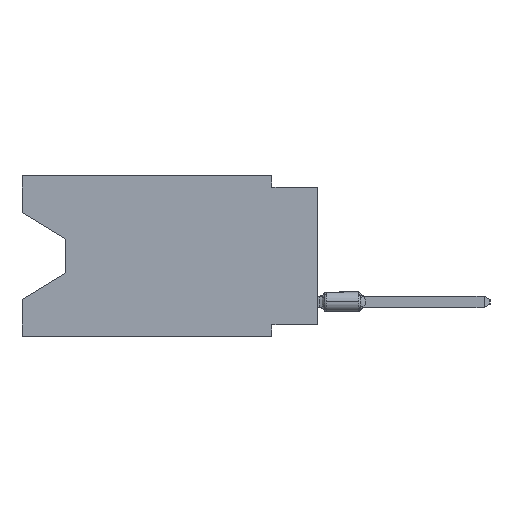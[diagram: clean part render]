
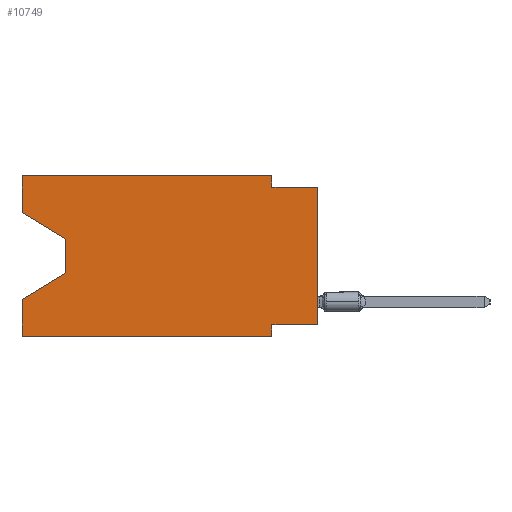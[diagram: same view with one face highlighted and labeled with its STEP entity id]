
A CAD part, left-side view. The second image highlights one B-rep face of the part: STEP entity #10749.
In plain terms, the highlighted planar face has unit normal (-1, 0, 0).
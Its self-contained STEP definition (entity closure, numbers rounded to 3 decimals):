
#308 = VERTEX_POINT ( 'NONE', #32423 ) ;
#1716 = ORIENTED_EDGE ( 'NONE', *, *, #21301, .T. ) ;
#2599 = VECTOR ( 'NONE', #13432, 1000. ) ;
#2848 = DIRECTION ( 'NONE',  ( 0., -1., 0. ) ) ;
#2854 = FACE_OUTER_BOUND ( 'NONE', #40116, .T. ) ;
#3252 = VERTEX_POINT ( 'NONE', #16704 ) ;
#3814 = CARTESIAN_POINT ( 'NONE',  ( 0., 2.54, -0.635 ) ) ;
#4680 = VECTOR ( 'NONE', #42543, 1000. ) ;
#5676 = VECTOR ( 'NONE', #6606, 1000. ) ;
#6606 = DIRECTION ( 'NONE',  ( 0., 0., -1. ) ) ;
#7299 = CARTESIAN_POINT ( 'NONE',  ( 0., 13.97, -3.505 ) ) ;
#7644 = CARTESIAN_POINT ( 'NONE',  ( 0., 16.383, 0. ) ) ;
#8144 = EDGE_CURVE ( 'NONE', #308, #26941, #40598, .T. ) ;
#8323 = CARTESIAN_POINT ( 'NONE',  ( 0., 16.383, -2.038 ) ) ;
#8617 = EDGE_CURVE ( 'NONE', #10358, #3252, #24710, .T. ) ;
#10027 = CARTESIAN_POINT ( 'NONE',  ( 0., 16.383, 0. ) ) ;
#10358 = VERTEX_POINT ( 'NONE', #16991 ) ;
#10749 = ADVANCED_FACE ( 'NONE', ( #2854 ), #16099, .F. ) ;
#10778 = LINE ( 'NONE', #16878, #35163 ) ;
#11109 = VECTOR ( 'NONE', #17625, 1000. ) ;
#11464 = ORIENTED_EDGE ( 'NONE', *, *, #41612, .F. ) ;
#11743 = VECTOR ( 'NONE', #32969, 1000. ) ;
#12427 = EDGE_CURVE ( 'NONE', #31995, #13780, #22536, .T. ) ;
#12822 = DIRECTION ( 'NONE',  ( 1., 0., 0. ) ) ;
#13432 = DIRECTION ( 'NONE',  ( 0., 1., 0. ) ) ;
#13780 = VERTEX_POINT ( 'NONE', #7299 ) ;
#14572 = ORIENTED_EDGE ( 'NONE', *, *, #26797, .T. ) ;
#15048 = LINE ( 'NONE', #21340, #22914 ) ;
#16099 = PLANE ( 'NONE',  #25712 ) ;
#16292 = CARTESIAN_POINT ( 'NONE',  ( 0., 16.383, -8.89 ) ) ;
#16387 = CARTESIAN_POINT ( 'NONE',  ( 0., 2.54, -8.89 ) ) ;
#16704 = CARTESIAN_POINT ( 'NONE',  ( 0., 16.383, -6.852 ) ) ;
#16878 = CARTESIAN_POINT ( 'NONE',  ( 0., 13.97, -5.385 ) ) ;
#16991 = CARTESIAN_POINT ( 'NONE',  ( 0., 16.383, -8.89 ) ) ;
#17625 = DIRECTION ( 'NONE',  ( 0., -1., 0. ) ) ;
#17955 = LINE ( 'NONE', #27698, #40091 ) ;
#18633 = VECTOR ( 'NONE', #34685, 1000. ) ;
#18640 = CARTESIAN_POINT ( 'NONE',  ( 0., 16.383, 0. ) ) ;
#19757 = LINE ( 'NONE', #16292, #11743 ) ;
#19933 = LINE ( 'NONE', #29273, #2599 ) ;
#20316 = CARTESIAN_POINT ( 'NONE',  ( 0., 0., -8.255 ) ) ;
#20758 = DIRECTION ( 'NONE',  ( 0., 0.855, -0.519 ) ) ;
#21301 = EDGE_CURVE ( 'NONE', #13780, #37296, #17955, .T. ) ;
#21340 = CARTESIAN_POINT ( 'NONE',  ( 0., 0., 0. ) ) ;
#21455 = CARTESIAN_POINT ( 'NONE',  ( 0., 2.54, 0. ) ) ;
#21619 = VERTEX_POINT ( 'NONE', #3814 ) ;
#22292 = VECTOR ( 'NONE', #35880, 1000. ) ;
#22536 = LINE ( 'NONE', #42030, #31858 ) ;
#22914 = VECTOR ( 'NONE', #34560, 1000. ) ;
#23104 = LINE ( 'NONE', #39782, #22292 ) ;
#23273 = EDGE_CURVE ( 'NONE', #30101, #32927, #23104, .T. ) ;
#24710 = LINE ( 'NONE', #18640, #18633 ) ;
#25712 = AXIS2_PLACEMENT_3D ( 'NONE', #29312, #12822, #26054 ) ;
#25946 = ORIENTED_EDGE ( 'NONE', *, *, #8617, .F. ) ;
#26054 = DIRECTION ( 'NONE',  ( 0., 0., -1. ) ) ;
#26562 = LINE ( 'NONE', #40206, #5676 ) ;
#26771 = EDGE_CURVE ( 'NONE', #21619, #27890, #36440, .T. ) ;
#26797 = EDGE_CURVE ( 'NONE', #10358, #32927, #19757, .T. ) ;
#26941 = VERTEX_POINT ( 'NONE', #21455 ) ;
#27295 = DIRECTION ( 'NONE',  ( 0., 0., -1. ) ) ;
#27652 = VECTOR ( 'NONE', #2848, 1000. ) ;
#27698 = CARTESIAN_POINT ( 'NONE',  ( 0., 13.97, -3.505 ) ) ;
#27809 = EDGE_CURVE ( 'NONE', #40372, #27890, #15048, .T. ) ;
#27890 = VERTEX_POINT ( 'NONE', #32612 ) ;
#29181 = ORIENTED_EDGE ( 'NONE', *, *, #12427, .T. ) ;
#29273 = CARTESIAN_POINT ( 'NONE',  ( 0., 0., -8.255 ) ) ;
#29312 = CARTESIAN_POINT ( 'NONE',  ( 0., 16.383, 0. ) ) ;
#29572 = ORIENTED_EDGE ( 'NONE', *, *, #27809, .T. ) ;
#29667 = ORIENTED_EDGE ( 'NONE', *, *, #40228, .F. ) ;
#29737 = ORIENTED_EDGE ( 'NONE', *, *, #8144, .F. ) ;
#30101 = VERTEX_POINT ( 'NONE', #35951 ) ;
#30134 = EDGE_CURVE ( 'NONE', #37296, #3252, #10778, .T. ) ;
#30141 = ORIENTED_EDGE ( 'NONE', *, *, #30134, .T. ) ;
#31787 = ORIENTED_EDGE ( 'NONE', *, *, #23273, .F. ) ;
#31858 = VECTOR ( 'NONE', #38794, 1000. ) ;
#31981 = CARTESIAN_POINT ( 'NONE',  ( 0., 13.97, -5.385 ) ) ;
#31995 = VERTEX_POINT ( 'NONE', #8323 ) ;
#32423 = CARTESIAN_POINT ( 'NONE',  ( 0., 16.383, 0. ) ) ;
#32612 = CARTESIAN_POINT ( 'NONE',  ( 0., 0., -0.635 ) ) ;
#32927 = VERTEX_POINT ( 'NONE', #16387 ) ;
#32969 = DIRECTION ( 'NONE',  ( 0., -1., 0. ) ) ;
#33688 = ORIENTED_EDGE ( 'NONE', *, *, #26771, .F. ) ;
#34560 = DIRECTION ( 'NONE',  ( 0., 0., 1. ) ) ;
#34685 = DIRECTION ( 'NONE',  ( 0., 0., 1. ) ) ;
#34999 = ORIENTED_EDGE ( 'NONE', *, *, #38636, .F. ) ;
#35163 = VECTOR ( 'NONE', #20758, 1000. ) ;
#35880 = DIRECTION ( 'NONE',  ( 0., 0., -1. ) ) ;
#35951 = CARTESIAN_POINT ( 'NONE',  ( 0., 2.54, -8.255 ) ) ;
#36012 = CARTESIAN_POINT ( 'NONE',  ( 0., 0., -0.635 ) ) ;
#36440 = LINE ( 'NONE', #36012, #27652 ) ;
#37296 = VERTEX_POINT ( 'NONE', #31981 ) ;
#38636 = EDGE_CURVE ( 'NONE', #26941, #21619, #26562, .T. ) ;
#38794 = DIRECTION ( 'NONE',  ( 0., -0.855, -0.519 ) ) ;
#39731 = LINE ( 'NONE', #10027, #4680 ) ;
#39782 = CARTESIAN_POINT ( 'NONE',  ( 0., 2.54, -8.89 ) ) ;
#40091 = VECTOR ( 'NONE', #27295, 1000. ) ;
#40116 = EDGE_LOOP ( 'NONE', ( #29181, #1716, #30141, #25946, #14572, #31787, #11464, #29572, #33688, #34999, #29737, #29667 ) ) ;
#40206 = CARTESIAN_POINT ( 'NONE',  ( 0., 2.54, 0. ) ) ;
#40228 = EDGE_CURVE ( 'NONE', #31995, #308, #39731, .T. ) ;
#40372 = VERTEX_POINT ( 'NONE', #20316 ) ;
#40598 = LINE ( 'NONE', #7644, #11109 ) ;
#41612 = EDGE_CURVE ( 'NONE', #40372, #30101, #19933, .T. ) ;
#42030 = CARTESIAN_POINT ( 'NONE',  ( 0., 16.383, -2.038 ) ) ;
#42543 = DIRECTION ( 'NONE',  ( 0., 0., 1. ) ) ;
